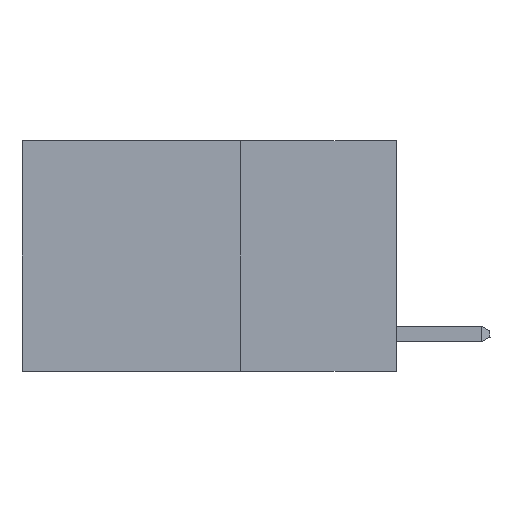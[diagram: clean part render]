
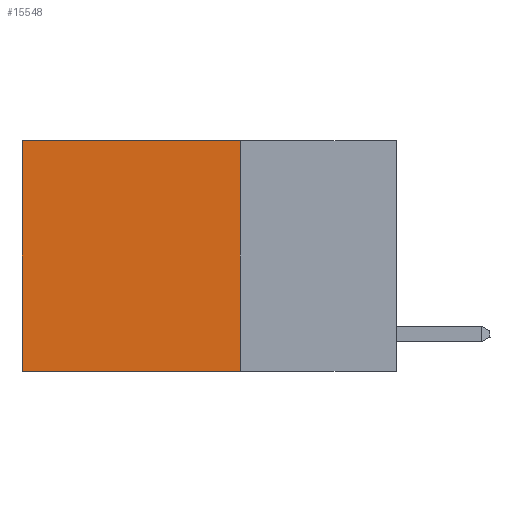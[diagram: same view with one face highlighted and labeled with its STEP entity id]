
A CAD part, left-side view. The second image highlights one B-rep face of the part: STEP entity #15548.
In plain terms, the highlighted planar face has unit normal (-1, 0, 0).
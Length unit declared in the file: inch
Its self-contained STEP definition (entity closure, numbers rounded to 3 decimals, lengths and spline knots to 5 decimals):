
#1283 = VERTEX_POINT ( 'NONE', #11919 ) ;
#1954 = DIRECTION ( 'NONE',  ( 0., 1., 0. ) ) ;
#2256 = VERTEX_POINT ( 'NONE', #14605 ) ;
#2891 = VECTOR ( 'NONE', #24962, 39.37008 ) ;
#3065 = ORIENTED_EDGE ( 'NONE', *, *, #23007, .T. ) ;
#3559 = EDGE_CURVE ( 'NONE', #2256, #25449, #5425, .T. ) ;
#4797 = FACE_OUTER_BOUND ( 'NONE', #8900, .T. ) ;
#4949 = VECTOR ( 'NONE', #1954, 39.37008 ) ;
#5425 = LINE ( 'NONE', #11211, #15259 ) ;
#6036 = CARTESIAN_POINT ( 'NONE',  ( 0.2625, 0.25, -0.37 ) ) ;
#6815 = VECTOR ( 'NONE', #23303, 39.37008 ) ;
#7660 = CARTESIAN_POINT ( 'NONE',  ( 0.2625, 0.6, 0. ) ) ;
#8900 = EDGE_LOOP ( 'NONE', ( #3065, #14173, #19395, #20592 ) ) ;
#8923 = PLANE ( 'NONE',  #18313 ) ;
#9265 = LINE ( 'NONE', #7660, #6815 ) ;
#10888 = DIRECTION ( 'NONE',  ( 1., 0., 0. ) ) ;
#11211 = CARTESIAN_POINT ( 'NONE',  ( 0.2625, 0.25, 0. ) ) ;
#11919 = CARTESIAN_POINT ( 'NONE',  ( 0.2625, 0.25, -0.37 ) ) ;
#13391 = LINE ( 'NONE', #15261, #2891 ) ;
#14173 = ORIENTED_EDGE ( 'NONE', *, *, #23132, .F. ) ;
#14362 = EDGE_CURVE ( 'NONE', #2256, #1283, #13391, .T. ) ;
#14605 = CARTESIAN_POINT ( 'NONE',  ( 0.2625, 0.25, 0. ) ) ;
#15160 = DIRECTION ( 'NONE',  ( 0., 1., 0. ) ) ;
#15259 = VECTOR ( 'NONE', #15160, 39.37008 ) ;
#15261 = CARTESIAN_POINT ( 'NONE',  ( 0.2625, 0.25, 0. ) ) ;
#15548 = ADVANCED_FACE ( 'NONE', ( #4797 ), #8923, .F. ) ;
#18313 = AXIS2_PLACEMENT_3D ( 'NONE', #22576, #10888, #24542 ) ;
#19364 = LINE ( 'NONE', #6036, #4949 ) ;
#19395 = ORIENTED_EDGE ( 'NONE', *, *, #14362, .F. ) ;
#20189 = VERTEX_POINT ( 'NONE', #24292 ) ;
#20592 = ORIENTED_EDGE ( 'NONE', *, *, #3559, .T. ) ;
#22027 = CARTESIAN_POINT ( 'NONE',  ( 0.2625, 0.6, 0. ) ) ;
#22576 = CARTESIAN_POINT ( 'NONE',  ( 0.2625, 0.25, 0. ) ) ;
#23007 = EDGE_CURVE ( 'NONE', #25449, #20189, #9265, .T. ) ;
#23132 = EDGE_CURVE ( 'NONE', #1283, #20189, #19364, .T. ) ;
#23303 = DIRECTION ( 'NONE',  ( 0., 0., -1. ) ) ;
#24292 = CARTESIAN_POINT ( 'NONE',  ( 0.2625, 0.6, -0.37 ) ) ;
#24542 = DIRECTION ( 'NONE',  ( 0., 0., -1. ) ) ;
#24962 = DIRECTION ( 'NONE',  ( 0., 0., -1. ) ) ;
#25449 = VERTEX_POINT ( 'NONE', #22027 ) ;
